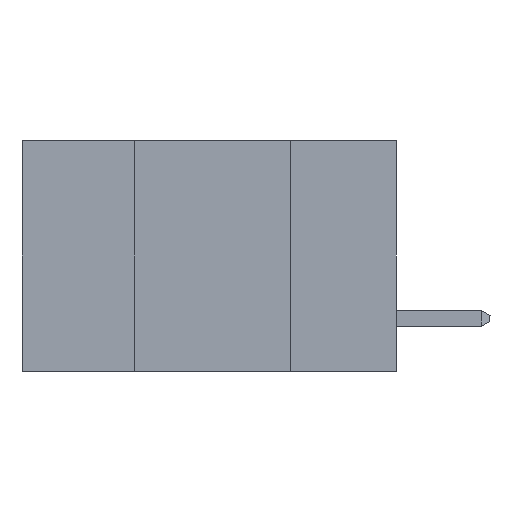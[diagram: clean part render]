
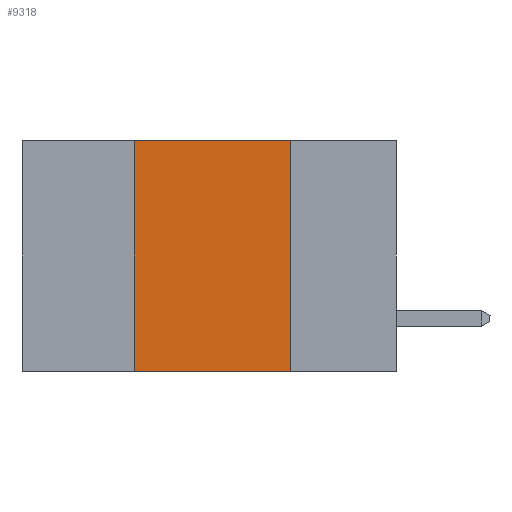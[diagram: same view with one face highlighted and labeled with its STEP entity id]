
A CAD part, left-side view. The second image highlights one B-rep face of the part: STEP entity #9318.
In plain terms, the highlighted planar face has unit normal (-1, 0, 0).
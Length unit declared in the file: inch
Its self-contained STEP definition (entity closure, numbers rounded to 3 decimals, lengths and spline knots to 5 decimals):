
#435 = ORIENTED_EDGE ( 'NONE', *, *, #1567, .T. ) ;
#465 = PLANE ( 'NONE',  #2504 ) ;
#641 = CARTESIAN_POINT ( 'NONE',  ( 0., 0.17, -0.37 ) ) ;
#1567 = EDGE_CURVE ( 'NONE', #14985, #14450, #12940, .T. ) ;
#1915 = VECTOR ( 'NONE', #6257, 39.37008 ) ;
#2363 = EDGE_CURVE ( 'NONE', #14985, #6529, #10239, .T. ) ;
#2504 = AXIS2_PLACEMENT_3D ( 'NONE', #6458, #2917, #11199 ) ;
#2589 = DIRECTION ( 'NONE',  ( 0., -1., 0. ) ) ;
#2720 = CARTESIAN_POINT ( 'NONE',  ( 0., 0.42, 0. ) ) ;
#2917 = DIRECTION ( 'NONE',  ( 1., 0., 0. ) ) ;
#3756 = ORIENTED_EDGE ( 'NONE', *, *, #5847, .F. ) ;
#4098 = VECTOR ( 'NONE', #8652, 39.37008 ) ;
#4695 = ORIENTED_EDGE ( 'NONE', *, *, #2363, .F. ) ;
#5562 = LINE ( 'NONE', #7392, #1915 ) ;
#5847 = EDGE_CURVE ( 'NONE', #6529, #7052, #5562, .T. ) ;
#6257 = DIRECTION ( 'NONE',  ( 0., -1., 0. ) ) ;
#6458 = CARTESIAN_POINT ( 'NONE',  ( 0., 0.6, 0. ) ) ;
#6529 = VERTEX_POINT ( 'NONE', #2720 ) ;
#6538 = FACE_OUTER_BOUND ( 'NONE', #9013, .T. ) ;
#6705 = VECTOR ( 'NONE', #14563, 39.37008 ) ;
#7052 = VERTEX_POINT ( 'NONE', #14177 ) ;
#7190 = LINE ( 'NONE', #7436, #4098 ) ;
#7392 = CARTESIAN_POINT ( 'NONE',  ( 0., 0.6, 0. ) ) ;
#7436 = CARTESIAN_POINT ( 'NONE',  ( 0., 0.17, -0.37 ) ) ;
#7838 = CARTESIAN_POINT ( 'NONE',  ( 0., 0.6, -0.37 ) ) ;
#8652 = DIRECTION ( 'NONE',  ( 0., 0., -1. ) ) ;
#9013 = EDGE_LOOP ( 'NONE', ( #13316, #3756, #4695, #435 ) ) ;
#9318 = ADVANCED_FACE ( 'NONE', ( #6538 ), #465, .F. ) ;
#10239 = LINE ( 'NONE', #11266, #6705 ) ;
#10273 = VECTOR ( 'NONE', #2589, 39.37008 ) ;
#11199 = DIRECTION ( 'NONE',  ( 0., 0., -1. ) ) ;
#11266 = CARTESIAN_POINT ( 'NONE',  ( 0., 0.42, -0.37 ) ) ;
#11618 = EDGE_CURVE ( 'NONE', #7052, #14450, #7190, .T. ) ;
#12940 = LINE ( 'NONE', #7838, #10273 ) ;
#13316 = ORIENTED_EDGE ( 'NONE', *, *, #11618, .F. ) ;
#14177 = CARTESIAN_POINT ( 'NONE',  ( 0., 0.17, 0. ) ) ;
#14450 = VERTEX_POINT ( 'NONE', #641 ) ;
#14563 = DIRECTION ( 'NONE',  ( 0., 0., 1. ) ) ;
#14985 = VERTEX_POINT ( 'NONE', #14996 ) ;
#14996 = CARTESIAN_POINT ( 'NONE',  ( 0., 0.42, -0.37 ) ) ;
